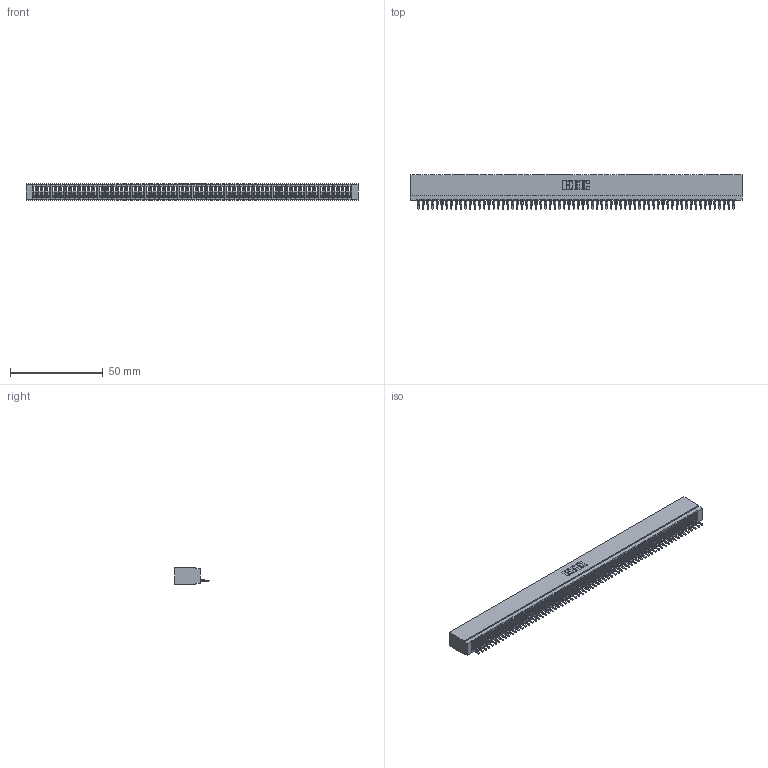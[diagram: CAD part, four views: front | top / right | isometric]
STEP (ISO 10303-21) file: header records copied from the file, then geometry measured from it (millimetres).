
FILE_DESCRIPTION (( 'STEP AP203' ), '1' );
FILE_NAME ('725-068-525-101.STEP', '2026-03-06T01:03:04', ( '' ), ( '' ), 'SwSTEP 2.0', 'SolidWorks 2023', '' );
FILE_SCHEMA (( 'CONFIG_CONTROL_DESIGN' ));
Length unit declared in the file: millimetre
Products named in the file (3): 725 Part_Insulator Option - 01; 745-292-001_525; 725-068-525-101
Assembly tree (69 placements, depth 2):
  725-068-525-101
    725 Part_Insulator Option - 01
    745-292-001_525  x68
Bounding box: 179.32 x 18.8 x 8.89 mm (x, y, z)
Volume: 13404.4 mm3; surface area: 26138.5 mm2
Topology: 69 solids, 69 shells, 7711 faces, 21198 edges, 13360 vertices
Faces by surface type: plane 4611, bspline 1360, cylinder 1332, torus 408
Entity records: 108718 total; most frequent: CARTESIAN_POINT 19659, ORIENTED_EDGE 19214, DIRECTION 16629, EDGE_CURVE 9607, LINE 9017, VECTOR 9017, VERTEX_POINT 6124, AXIS2_PLACEMENT_3D 3806
